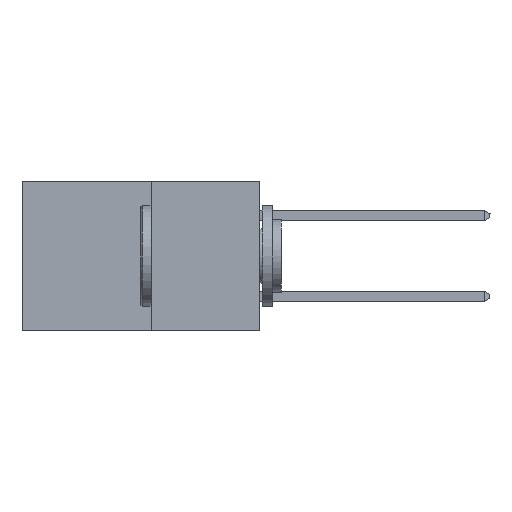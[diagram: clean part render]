
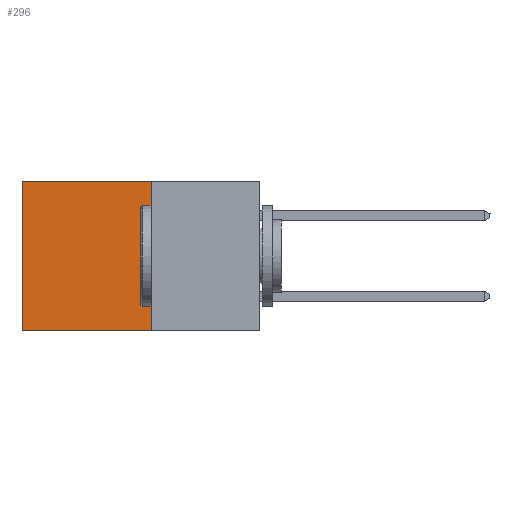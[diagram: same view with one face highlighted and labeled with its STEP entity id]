
A CAD part, left-side view. The second image highlights one B-rep face of the part: STEP entity #296.
In plain terms, the highlighted planar face has unit normal (-1, 0, 0).
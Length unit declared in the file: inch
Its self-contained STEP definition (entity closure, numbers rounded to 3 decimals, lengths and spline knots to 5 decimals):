
#26 = EDGE_LOOP ( 'NONE', ( #3478, #3088, #2489, #1033 ) ) ;
#65 = EDGE_CURVE ( 'NONE', #7639, #4489, #5922, .T. ) ;
#135 = CARTESIAN_POINT ( 'NONE',  ( 0.277, 0.59, -0.37 ) ) ;
#156 = VERTEX_POINT ( 'NONE', #8461 ) ;
#242 = DIRECTION ( 'NONE',  ( 0., 1., 0. ) ) ;
#296 = ADVANCED_FACE ( 'NONE', ( #1794 ), #9211, .F. ) ;
#567 = CARTESIAN_POINT ( 'NONE',  ( 0.277, 0.27, 0. ) ) ;
#855 = CARTESIAN_POINT ( 'NONE',  ( 0.277, 0.27, -0.37 ) ) ;
#947 = VECTOR ( 'NONE', #242, 39.37008 ) ;
#1033 = ORIENTED_EDGE ( 'NONE', *, *, #6664, .T. ) ;
#1051 = LINE ( 'NONE', #855, #6859 ) ;
#1749 = CARTESIAN_POINT ( 'NONE',  ( 0.277, 0.59, 0. ) ) ;
#1794 = FACE_OUTER_BOUND ( 'NONE', #26, .T. ) ;
#1830 = CARTESIAN_POINT ( 'NONE',  ( 0.277, 0.59, -0.37 ) ) ;
#2119 = DIRECTION ( 'NONE',  ( 0., 1., 0. ) ) ;
#2419 = DIRECTION ( 'NONE',  ( 0., 0., -1. ) ) ;
#2489 = ORIENTED_EDGE ( 'NONE', *, *, #9545, .F. ) ;
#3088 = ORIENTED_EDGE ( 'NONE', *, *, #8799, .F. ) ;
#3260 = LINE ( 'NONE', #9578, #947 ) ;
#3478 = ORIENTED_EDGE ( 'NONE', *, *, #65, .T. ) ;
#4489 = VERTEX_POINT ( 'NONE', #1830 ) ;
#5867 = CARTESIAN_POINT ( 'NONE',  ( 0.277, 0.27, -0.37 ) ) ;
#5922 = LINE ( 'NONE', #135, #9479 ) ;
#6061 = DIRECTION ( 'NONE',  ( 0., 0., -1. ) ) ;
#6664 = EDGE_CURVE ( 'NONE', #7786, #7639, #3260, .T. ) ;
#6740 = VECTOR ( 'NONE', #2119, 39.37008 ) ;
#6859 = VECTOR ( 'NONE', #2419, 39.37008 ) ;
#7297 = AXIS2_PLACEMENT_3D ( 'NONE', #7366, #9254, #9345 ) ;
#7366 = CARTESIAN_POINT ( 'NONE',  ( 0.277, 0.27, -0.37 ) ) ;
#7639 = VERTEX_POINT ( 'NONE', #1749 ) ;
#7786 = VERTEX_POINT ( 'NONE', #567 ) ;
#8461 = CARTESIAN_POINT ( 'NONE',  ( 0.277, 0.27, -0.37 ) ) ;
#8644 = LINE ( 'NONE', #5867, #6740 ) ;
#8799 = EDGE_CURVE ( 'NONE', #156, #4489, #8644, .T. ) ;
#9211 = PLANE ( 'NONE',  #7297 ) ;
#9254 = DIRECTION ( 'NONE',  ( 1., 0., 0. ) ) ;
#9345 = DIRECTION ( 'NONE',  ( 0., 0., -1. ) ) ;
#9479 = VECTOR ( 'NONE', #6061, 39.37008 ) ;
#9545 = EDGE_CURVE ( 'NONE', #7786, #156, #1051, .T. ) ;
#9578 = CARTESIAN_POINT ( 'NONE',  ( 0.277, 0.27, 0. ) ) ;
